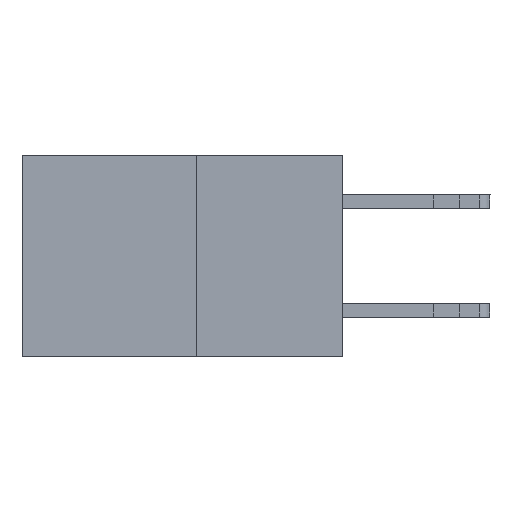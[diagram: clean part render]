
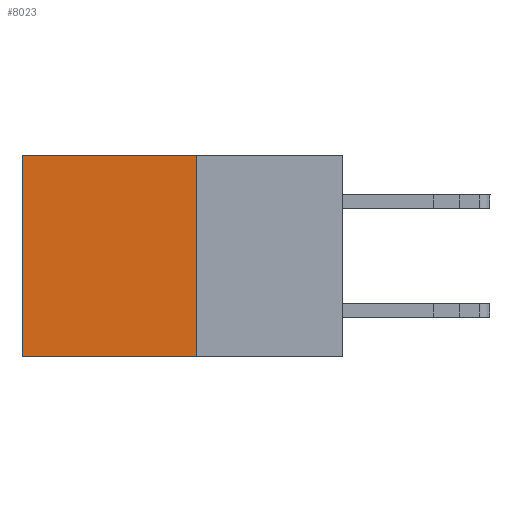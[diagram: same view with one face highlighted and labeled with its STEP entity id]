
A CAD part, left-side view. The second image highlights one B-rep face of the part: STEP entity #8023.
In plain terms, the highlighted planar face has unit normal (-1, 0, 0).
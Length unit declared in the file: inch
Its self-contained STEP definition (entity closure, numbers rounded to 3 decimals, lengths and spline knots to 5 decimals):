
#427 = AXIS2_PLACEMENT_3D ( 'NONE', #4511, #4042, #3860 ) ;
#471 = ORIENTED_EDGE ( 'NONE', *, *, #581, .F. ) ;
#581 = EDGE_CURVE ( 'NONE', #1051, #7383, #4278, .T. ) ;
#1051 = VERTEX_POINT ( 'NONE', #3832 ) ;
#1368 = EDGE_LOOP ( 'NONE', ( #8790, #471, #3671, #11849 ) ) ;
#2703 = EDGE_CURVE ( 'NONE', #10450, #7383, #5272, .T. ) ;
#3671 = ORIENTED_EDGE ( 'NONE', *, *, #8518, .F. ) ;
#3832 = CARTESIAN_POINT ( 'NONE',  ( 0.277, 0.27, -0.37 ) ) ;
#3860 = DIRECTION ( 'NONE',  ( 0., 0., -1. ) ) ;
#4042 = DIRECTION ( 'NONE',  ( 1., 0., 0. ) ) ;
#4123 = CARTESIAN_POINT ( 'NONE',  ( 0.277, 0.59, -0.37 ) ) ;
#4278 = LINE ( 'NONE', #8286, #9877 ) ;
#4311 = PLANE ( 'NONE',  #427 ) ;
#4511 = CARTESIAN_POINT ( 'NONE',  ( 0.277, 0.27, -0.37 ) ) ;
#5272 = LINE ( 'NONE', #4123, #10830 ) ;
#5303 = DIRECTION ( 'NONE',  ( 0., 0., -1. ) ) ;
#6685 = VERTEX_POINT ( 'NONE', #12466 ) ;
#7383 = VERTEX_POINT ( 'NONE', #10780 ) ;
#8023 = ADVANCED_FACE ( 'NONE', ( #11387 ), #4311, .F. ) ;
#8286 = CARTESIAN_POINT ( 'NONE',  ( 0.277, 0.27, -0.37 ) ) ;
#8518 = EDGE_CURVE ( 'NONE', #6685, #1051, #14588, .T. ) ;
#8597 = CARTESIAN_POINT ( 'NONE',  ( 0.277, 0.59, 0. ) ) ;
#8790 = ORIENTED_EDGE ( 'NONE', *, *, #2703, .T. ) ;
#9605 = DIRECTION ( 'NONE',  ( 0., 1., 0. ) ) ;
#9877 = VECTOR ( 'NONE', #13766, 39.37008 ) ;
#9961 = VECTOR ( 'NONE', #9605, 39.37008 ) ;
#10450 = VERTEX_POINT ( 'NONE', #8597 ) ;
#10780 = CARTESIAN_POINT ( 'NONE',  ( 0.277, 0.59, -0.37 ) ) ;
#10830 = VECTOR ( 'NONE', #12309, 39.37008 ) ;
#11106 = EDGE_CURVE ( 'NONE', #6685, #10450, #12855, .T. ) ;
#11387 = FACE_OUTER_BOUND ( 'NONE', #1368, .T. ) ;
#11708 = VECTOR ( 'NONE', #5303, 39.37008 ) ;
#11849 = ORIENTED_EDGE ( 'NONE', *, *, #11106, .T. ) ;
#12309 = DIRECTION ( 'NONE',  ( 0., 0., -1. ) ) ;
#12466 = CARTESIAN_POINT ( 'NONE',  ( 0.277, 0.27, 0. ) ) ;
#12843 = CARTESIAN_POINT ( 'NONE',  ( 0.277, 0.27, 0. ) ) ;
#12855 = LINE ( 'NONE', #12843, #9961 ) ;
#13057 = CARTESIAN_POINT ( 'NONE',  ( 0.277, 0.27, -0.37 ) ) ;
#13766 = DIRECTION ( 'NONE',  ( 0., 1., 0. ) ) ;
#14588 = LINE ( 'NONE', #13057, #11708 ) ;
